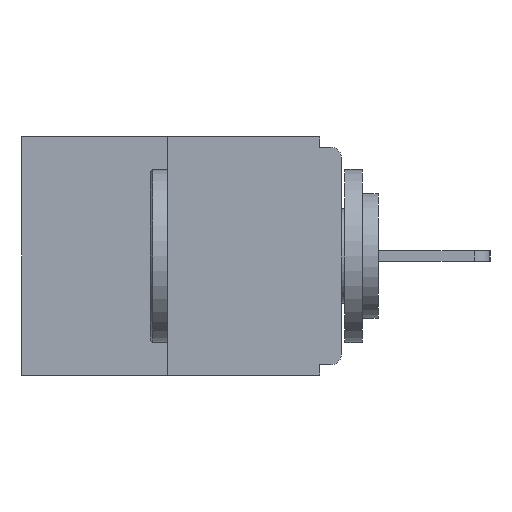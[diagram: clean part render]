
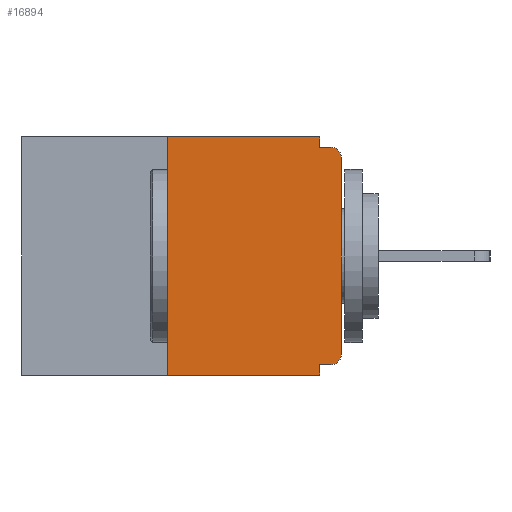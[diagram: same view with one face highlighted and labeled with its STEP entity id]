
A CAD part, left-side view. The second image highlights one B-rep face of the part: STEP entity #16894.
In plain terms, the highlighted planar face has unit normal (-1, 0, 0).
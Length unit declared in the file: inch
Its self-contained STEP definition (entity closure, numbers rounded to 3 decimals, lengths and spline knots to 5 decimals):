
#192 = CARTESIAN_POINT ( 'NONE',  ( 0., 0., 0. ) ) ;
#306 = VECTOR ( 'NONE', #13848, 39.37008 ) ;
#748 = VECTOR ( 'NONE', #12777, 39.37008 ) ;
#935 = CIRCLE ( 'NONE', #1664, 0.015 ) ;
#962 = VECTOR ( 'NONE', #3200, 39.37008 ) ;
#1255 = CARTESIAN_POINT ( 'NONE',  ( 0., 0., -0.03 ) ) ;
#1258 = DIRECTION ( 'NONE',  ( 0., 0., -1. ) ) ;
#1392 = AXIS2_PLACEMENT_3D ( 'NONE', #8332, #21515, #10261 ) ;
#1575 = LINE ( 'NONE', #7133, #962 ) ;
#1664 = AXIS2_PLACEMENT_3D ( 'NONE', #20263, #20203, #20100 ) ;
#2173 = DIRECTION ( 'NONE',  ( 0., 0., 1. ) ) ;
#2518 = EDGE_CURVE ( 'NONE', #17284, #5565, #4109, .T. ) ;
#2647 = LINE ( 'NONE', #9070, #17409 ) ;
#3194 = CARTESIAN_POINT ( 'NONE',  ( 0., 0.031, -0.343 ) ) ;
#3200 = DIRECTION ( 'NONE',  ( 0., -1., 0. ) ) ;
#3823 = EDGE_CURVE ( 'NONE', #22729, #17516, #935, .T. ) ;
#4109 = LINE ( 'NONE', #13167, #23268 ) ;
#4887 = CARTESIAN_POINT ( 'NONE',  ( 0., 0.031, -0.015 ) ) ;
#5149 = DIRECTION ( 'NONE',  ( 0., -1., 0. ) ) ;
#5271 = CARTESIAN_POINT ( 'NONE',  ( 0., 0.031, -0.343 ) ) ;
#5540 = AXIS2_PLACEMENT_3D ( 'NONE', #23947, #6914, #20193 ) ;
#5565 = VERTEX_POINT ( 'NONE', #23525 ) ;
#5675 = ORIENTED_EDGE ( 'NONE', *, *, #2518, .F. ) ;
#6017 = LINE ( 'NONE', #16465, #748 ) ;
#6543 = EDGE_LOOP ( 'NONE', ( #5675, #16463, #21473, #7579, #12651, #17618, #8802, #24479, #15034, #20612 ) ) ;
#6879 = VERTEX_POINT ( 'NONE', #16621 ) ;
#6914 = DIRECTION ( 'NONE',  ( 1., 0., 0. ) ) ;
#7133 = CARTESIAN_POINT ( 'NONE',  ( 0., 0.46, -0.343 ) ) ;
#7579 = ORIENTED_EDGE ( 'NONE', *, *, #18901, .F. ) ;
#7714 = CARTESIAN_POINT ( 'NONE',  ( 0., 0.031, -0.328 ) ) ;
#7856 = EDGE_CURVE ( 'NONE', #6879, #8285, #13479, .T. ) ;
#8285 = VERTEX_POINT ( 'NONE', #9584 ) ;
#8315 = VECTOR ( 'NONE', #16911, 39.37008 ) ;
#8332 = CARTESIAN_POINT ( 'NONE',  ( 0., 0.015, -0.313 ) ) ;
#8802 = ORIENTED_EDGE ( 'NONE', *, *, #24344, .T. ) ;
#9070 = CARTESIAN_POINT ( 'NONE',  ( 0., 0.031, 0. ) ) ;
#9584 = CARTESIAN_POINT ( 'NONE',  ( 0., 0., -0.313 ) ) ;
#10261 = DIRECTION ( 'NONE',  ( 0., 0., -1. ) ) ;
#10431 = EDGE_CURVE ( 'NONE', #13719, #17516, #18314, .T. ) ;
#10963 = DIRECTION ( 'NONE',  ( 0., 0., -1. ) ) ;
#11958 = CARTESIAN_POINT ( 'NONE',  ( 0., 0., -0.328 ) ) ;
#12131 = VERTEX_POINT ( 'NONE', #3194 ) ;
#12651 = ORIENTED_EDGE ( 'NONE', *, *, #15469, .F. ) ;
#12777 = DIRECTION ( 'NONE',  ( 0., 0., 1. ) ) ;
#13167 = CARTESIAN_POINT ( 'NONE',  ( 0., 0.46, 0. ) ) ;
#13479 = CIRCLE ( 'NONE', #1392, 0.015 ) ;
#13719 = VERTEX_POINT ( 'NONE', #4887 ) ;
#13848 = DIRECTION ( 'NONE',  ( 0., 1., 0. ) ) ;
#14045 = LINE ( 'NONE', #192, #23502 ) ;
#15034 = ORIENTED_EDGE ( 'NONE', *, *, #10431, .F. ) ;
#15062 = CARTESIAN_POINT ( 'NONE',  ( 0., 0., -0.015 ) ) ;
#15305 = VERTEX_POINT ( 'NONE', #7714 ) ;
#15469 = EDGE_CURVE ( 'NONE', #6879, #15305, #15774, .T. ) ;
#15581 = CARTESIAN_POINT ( 'NONE',  ( 0., 0.25, 0. ) ) ;
#15774 = LINE ( 'NONE', #11958, #306 ) ;
#16405 = PLANE ( 'NONE',  #5540 ) ;
#16463 = ORIENTED_EDGE ( 'NONE', *, *, #21437, .F. ) ;
#16465 = CARTESIAN_POINT ( 'NONE',  ( 0., 0.25, 0. ) ) ;
#16621 = CARTESIAN_POINT ( 'NONE',  ( 0., 0.015, -0.328 ) ) ;
#16894 = ADVANCED_FACE ( 'NONE', ( #23400 ), #16405, .F. ) ;
#16911 = DIRECTION ( 'NONE',  ( 0., -1., 0. ) ) ;
#17284 = VERTEX_POINT ( 'NONE', #15581 ) ;
#17409 = VECTOR ( 'NONE', #10963, 39.37008 ) ;
#17516 = VERTEX_POINT ( 'NONE', #18088 ) ;
#17618 = ORIENTED_EDGE ( 'NONE', *, *, #7856, .T. ) ;
#17628 = EDGE_CURVE ( 'NONE', #5565, #13719, #2647, .T. ) ;
#17907 = VERTEX_POINT ( 'NONE', #21142 ) ;
#18088 = CARTESIAN_POINT ( 'NONE',  ( 0., 0.015, -0.015 ) ) ;
#18314 = LINE ( 'NONE', #15062, #8315 ) ;
#18901 = EDGE_CURVE ( 'NONE', #15305, #12131, #19099, .T. ) ;
#19099 = LINE ( 'NONE', #5271, #23583 ) ;
#20100 = DIRECTION ( 'NONE',  ( 0., 0., -1. ) ) ;
#20178 = EDGE_CURVE ( 'NONE', #17907, #12131, #1575, .T. ) ;
#20193 = DIRECTION ( 'NONE',  ( 0., 0., -1. ) ) ;
#20203 = DIRECTION ( 'NONE',  ( -1., 0., 0. ) ) ;
#20263 = CARTESIAN_POINT ( 'NONE',  ( 0., 0.015, -0.03 ) ) ;
#20612 = ORIENTED_EDGE ( 'NONE', *, *, #17628, .F. ) ;
#21142 = CARTESIAN_POINT ( 'NONE',  ( 0., 0.25, -0.343 ) ) ;
#21437 = EDGE_CURVE ( 'NONE', #17907, #17284, #6017, .T. ) ;
#21473 = ORIENTED_EDGE ( 'NONE', *, *, #20178, .T. ) ;
#21515 = DIRECTION ( 'NONE',  ( -1., 0., 0. ) ) ;
#22729 = VERTEX_POINT ( 'NONE', #1255 ) ;
#23268 = VECTOR ( 'NONE', #5149, 39.37008 ) ;
#23400 = FACE_OUTER_BOUND ( 'NONE', #6543, .T. ) ;
#23502 = VECTOR ( 'NONE', #2173, 39.37008 ) ;
#23525 = CARTESIAN_POINT ( 'NONE',  ( 0., 0.031, 0. ) ) ;
#23583 = VECTOR ( 'NONE', #1258, 39.37008 ) ;
#23947 = CARTESIAN_POINT ( 'NONE',  ( 0., 0.46, 0. ) ) ;
#24344 = EDGE_CURVE ( 'NONE', #8285, #22729, #14045, .T. ) ;
#24479 = ORIENTED_EDGE ( 'NONE', *, *, #3823, .T. ) ;
